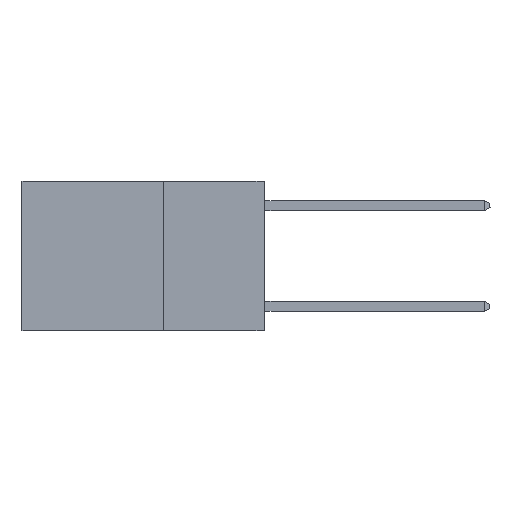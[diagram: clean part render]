
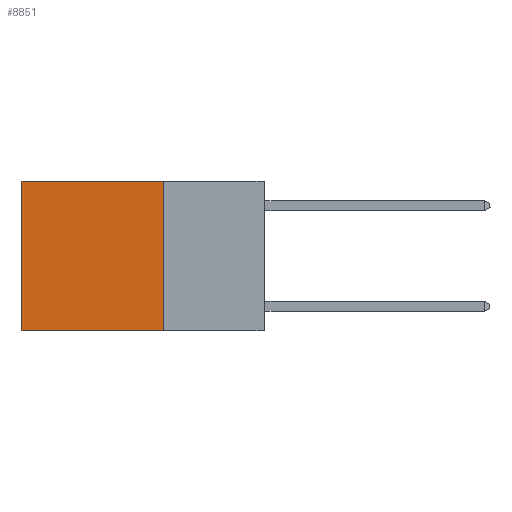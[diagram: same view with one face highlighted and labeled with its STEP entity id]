
A CAD part, left-side view. The second image highlights one B-rep face of the part: STEP entity #8851.
In plain terms, the highlighted planar face has unit normal (-1, 0, 0).
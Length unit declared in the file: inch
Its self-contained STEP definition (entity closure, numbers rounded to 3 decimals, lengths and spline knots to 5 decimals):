
#51 = VECTOR ( 'NONE', #12495, 39.37008 ) ;
#414 = AXIS2_PLACEMENT_3D ( 'NONE', #12252, #13390, #6362 ) ;
#565 = ORIENTED_EDGE ( 'NONE', *, *, #6763, .F. ) ;
#1070 = LINE ( 'NONE', #11086, #8102 ) ;
#1305 = ORIENTED_EDGE ( 'NONE', *, *, #8308, .T. ) ;
#1829 = CARTESIAN_POINT ( 'NONE',  ( 0.2625, 0.25, 0. ) ) ;
#1956 = ORIENTED_EDGE ( 'NONE', *, *, #8085, .T. ) ;
#2076 = CARTESIAN_POINT ( 'NONE',  ( 0.2625, 0.6, 0. ) ) ;
#2300 = FACE_OUTER_BOUND ( 'NONE', #13203, .T. ) ;
#2383 = LINE ( 'NONE', #4180, #51 ) ;
#2790 = DIRECTION ( 'NONE',  ( 0., 1., 0. ) ) ;
#3209 = VECTOR ( 'NONE', #10482, 39.37008 ) ;
#3321 = CARTESIAN_POINT ( 'NONE',  ( 0.2625, 0.6, 0. ) ) ;
#3943 = PLANE ( 'NONE',  #414 ) ;
#4180 = CARTESIAN_POINT ( 'NONE',  ( 0.2625, 0.25, -0.37 ) ) ;
#4232 = ORIENTED_EDGE ( 'NONE', *, *, #8918, .F. ) ;
#5734 = CARTESIAN_POINT ( 'NONE',  ( 0.2625, 0.25, 0. ) ) ;
#6362 = DIRECTION ( 'NONE',  ( 0., 0., -1. ) ) ;
#6735 = LINE ( 'NONE', #3321, #3209 ) ;
#6763 = EDGE_CURVE ( 'NONE', #8199, #11922, #2383, .T. ) ;
#7847 = CARTESIAN_POINT ( 'NONE',  ( 0.2625, 0.25, -0.37 ) ) ;
#7854 = VERTEX_POINT ( 'NONE', #5734 ) ;
#8085 = EDGE_CURVE ( 'NONE', #7854, #12354, #1070, .T. ) ;
#8102 = VECTOR ( 'NONE', #2790, 39.37008 ) ;
#8199 = VERTEX_POINT ( 'NONE', #7847 ) ;
#8308 = EDGE_CURVE ( 'NONE', #12354, #11922, #6735, .T. ) ;
#8486 = CARTESIAN_POINT ( 'NONE',  ( 0.2625, 0.6, -0.37 ) ) ;
#8851 = ADVANCED_FACE ( 'NONE', ( #2300 ), #3943, .F. ) ;
#8918 = EDGE_CURVE ( 'NONE', #7854, #8199, #13154, .T. ) ;
#10482 = DIRECTION ( 'NONE',  ( 0., 0., -1. ) ) ;
#11086 = CARTESIAN_POINT ( 'NONE',  ( 0.2625, 0.25, 0. ) ) ;
#11922 = VERTEX_POINT ( 'NONE', #8486 ) ;
#12252 = CARTESIAN_POINT ( 'NONE',  ( 0.2625, 0.25, 0. ) ) ;
#12354 = VERTEX_POINT ( 'NONE', #2076 ) ;
#12495 = DIRECTION ( 'NONE',  ( 0., 1., 0. ) ) ;
#13154 = LINE ( 'NONE', #1829, #13858 ) ;
#13203 = EDGE_LOOP ( 'NONE', ( #1305, #565, #4232, #1956 ) ) ;
#13390 = DIRECTION ( 'NONE',  ( 1., 0., 0. ) ) ;
#13540 = DIRECTION ( 'NONE',  ( 0., 0., -1. ) ) ;
#13858 = VECTOR ( 'NONE', #13540, 39.37008 ) ;
